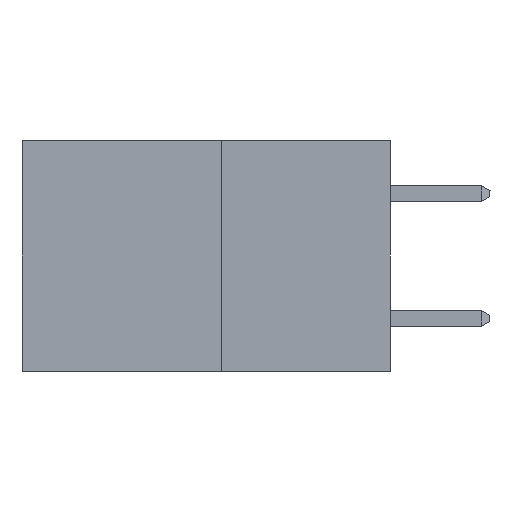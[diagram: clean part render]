
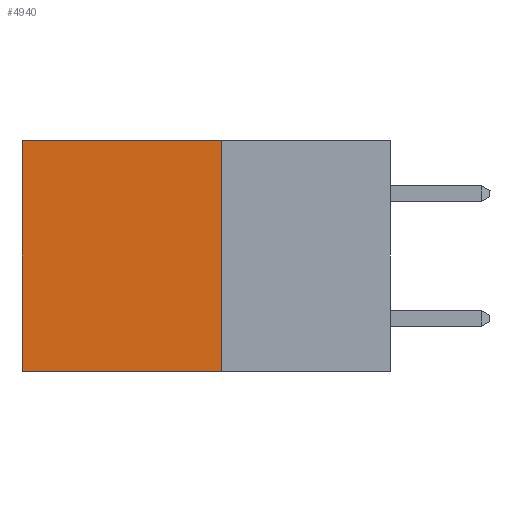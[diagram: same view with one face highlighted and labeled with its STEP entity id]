
A CAD part, left-side view. The second image highlights one B-rep face of the part: STEP entity #4940.
In plain terms, the highlighted planar face has unit normal (-1, 0, 0).
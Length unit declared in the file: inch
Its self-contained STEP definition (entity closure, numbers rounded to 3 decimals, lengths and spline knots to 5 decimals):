
#505 = VERTEX_POINT ( 'NONE', #5227 ) ;
#681 = DIRECTION ( 'NONE',  ( 0., 0., -1. ) ) ;
#775 = VERTEX_POINT ( 'NONE', #10064 ) ;
#1067 = CARTESIAN_POINT ( 'NONE',  ( 0.277, 0.27, -0.37 ) ) ;
#1159 = ORIENTED_EDGE ( 'NONE', *, *, #5587, .F. ) ;
#1929 = EDGE_CURVE ( 'NONE', #505, #9758, #5396, .T. ) ;
#2100 = VECTOR ( 'NONE', #8309, 39.37008 ) ;
#2294 = EDGE_CURVE ( 'NONE', #2957, #775, #11481, .T. ) ;
#2957 = VERTEX_POINT ( 'NONE', #8378 ) ;
#3221 = CARTESIAN_POINT ( 'NONE',  ( 0.277, 0.59, -0.37 ) ) ;
#3982 = CARTESIAN_POINT ( 'NONE',  ( 0.277, 0.59, 0. ) ) ;
#4369 = PLANE ( 'NONE',  #11362 ) ;
#4940 = ADVANCED_FACE ( 'NONE', ( #5612 ), #4369, .F. ) ;
#5077 = DIRECTION ( 'NONE',  ( 0., 1., 0. ) ) ;
#5227 = CARTESIAN_POINT ( 'NONE',  ( 0.277, 0.27, 0. ) ) ;
#5317 = CARTESIAN_POINT ( 'NONE',  ( 0.277, 0.27, -0.37 ) ) ;
#5396 = LINE ( 'NONE', #8593, #9751 ) ;
#5419 = CARTESIAN_POINT ( 'NONE',  ( 0.277, 0.27, -0.37 ) ) ;
#5587 = EDGE_CURVE ( 'NONE', #505, #2957, #6028, .T. ) ;
#5612 = FACE_OUTER_BOUND ( 'NONE', #6335, .T. ) ;
#6028 = LINE ( 'NONE', #5419, #10373 ) ;
#6209 = DIRECTION ( 'NONE',  ( 1., 0., 0. ) ) ;
#6335 = EDGE_LOOP ( 'NONE', ( #10821, #9553, #1159, #8376 ) ) ;
#6740 = EDGE_CURVE ( 'NONE', #9758, #775, #8754, .T. ) ;
#8309 = DIRECTION ( 'NONE',  ( 0., 1., 0. ) ) ;
#8376 = ORIENTED_EDGE ( 'NONE', *, *, #1929, .T. ) ;
#8378 = CARTESIAN_POINT ( 'NONE',  ( 0.277, 0.27, -0.37 ) ) ;
#8593 = CARTESIAN_POINT ( 'NONE',  ( 0.277, 0.27, 0. ) ) ;
#8754 = LINE ( 'NONE', #3221, #11272 ) ;
#8947 = DIRECTION ( 'NONE',  ( 0., 0., -1. ) ) ;
#9441 = DIRECTION ( 'NONE',  ( 0., 0., -1. ) ) ;
#9553 = ORIENTED_EDGE ( 'NONE', *, *, #2294, .F. ) ;
#9751 = VECTOR ( 'NONE', #5077, 39.37008 ) ;
#9758 = VERTEX_POINT ( 'NONE', #3982 ) ;
#10064 = CARTESIAN_POINT ( 'NONE',  ( 0.277, 0.59, -0.37 ) ) ;
#10373 = VECTOR ( 'NONE', #8947, 39.37008 ) ;
#10821 = ORIENTED_EDGE ( 'NONE', *, *, #6740, .T. ) ;
#11272 = VECTOR ( 'NONE', #9441, 39.37008 ) ;
#11362 = AXIS2_PLACEMENT_3D ( 'NONE', #5317, #6209, #681 ) ;
#11481 = LINE ( 'NONE', #1067, #2100 ) ;
